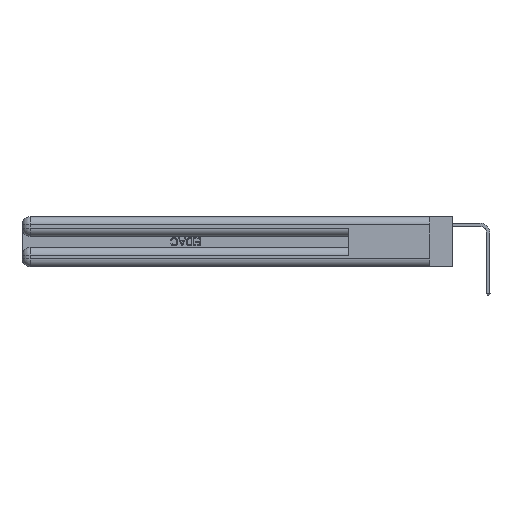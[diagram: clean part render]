
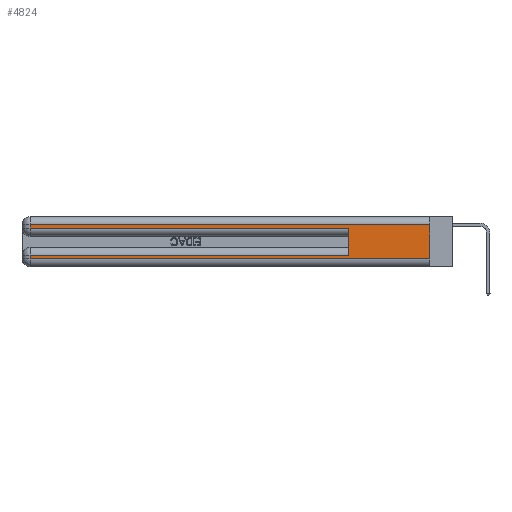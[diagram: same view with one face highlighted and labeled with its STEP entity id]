
A CAD part, left-side view. The second image highlights one B-rep face of the part: STEP entity #4824.
In plain terms, the highlighted planar face has unit normal (-1, 0, 0).
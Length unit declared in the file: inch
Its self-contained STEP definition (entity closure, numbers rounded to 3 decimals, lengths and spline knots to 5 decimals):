
#59 = VECTOR ( 'NONE', #2766, 39.37008 ) ;
#633 = CARTESIAN_POINT ( 'NONE',  ( 0., 0., 0.37 ) ) ;
#1329 = CARTESIAN_POINT ( 'NONE',  ( 0., 0.6, 0.285 ) ) ;
#1531 = VERTEX_POINT ( 'NONE', #12219 ) ;
#1656 = LINE ( 'NONE', #18666, #21440 ) ;
#1940 = DIRECTION ( 'NONE',  ( 0., 0., -1. ) ) ;
#2124 = DIRECTION ( 'NONE',  ( 0., -1., 0. ) ) ;
#2766 = DIRECTION ( 'NONE',  ( 0., 0., -1. ) ) ;
#2821 = CARTESIAN_POINT ( 'NONE',  ( 0., 0., 0.37 ) ) ;
#2968 = DIRECTION ( 'NONE',  ( 0., 0., -1. ) ) ;
#3170 = ORIENTED_EDGE ( 'NONE', *, *, #26253, .T. ) ;
#3863 = DIRECTION ( 'NONE',  ( 0., -1., 0. ) ) ;
#4611 = CARTESIAN_POINT ( 'NONE',  ( 0., 0.6, 0.085 ) ) ;
#4824 = ADVANCED_FACE ( 'NONE', ( #29267 ), #7460, .F. ) ;
#4844 = EDGE_CURVE ( 'NONE', #19728, #23056, #17639, .T. ) ;
#5137 = CARTESIAN_POINT ( 'NONE',  ( 0., 2.94, 0.37 ) ) ;
#5195 = LINE ( 'NONE', #2821, #23765 ) ;
#5652 = CARTESIAN_POINT ( 'NONE',  ( 0., 2.94, 0.06 ) ) ;
#7460 = PLANE ( 'NONE',  #13780 ) ;
#9401 = CARTESIAN_POINT ( 'NONE',  ( 0., 2.94, 0.37 ) ) ;
#9606 = LINE ( 'NONE', #11847, #10082 ) ;
#10082 = VECTOR ( 'NONE', #17260, 39.37008 ) ;
#10135 = VECTOR ( 'NONE', #11826, 39.37008 ) ;
#11091 = EDGE_CURVE ( 'NONE', #17404, #16599, #14023, .T. ) ;
#11424 = CARTESIAN_POINT ( 'NONE',  ( 0., 0., 0.31 ) ) ;
#11826 = DIRECTION ( 'NONE',  ( 0., 0., 1. ) ) ;
#11847 = CARTESIAN_POINT ( 'NONE',  ( 0., 0., 0.085 ) ) ;
#12061 = ORIENTED_EDGE ( 'NONE', *, *, #11091, .T. ) ;
#12219 = CARTESIAN_POINT ( 'NONE',  ( 0., 2.94, 0.285 ) ) ;
#12253 = ORIENTED_EDGE ( 'NONE', *, *, #23209, .T. ) ;
#12267 = ORIENTED_EDGE ( 'NONE', *, *, #4844, .T. ) ;
#12550 = DIRECTION ( 'NONE',  ( 0., 1., 0. ) ) ;
#13015 = DIRECTION ( 'NONE',  ( 1., 0., 0. ) ) ;
#13780 = AXIS2_PLACEMENT_3D ( 'NONE', #633, #13015, #27194 ) ;
#14023 = LINE ( 'NONE', #9401, #26187 ) ;
#14520 = LINE ( 'NONE', #21853, #10135 ) ;
#15435 = CARTESIAN_POINT ( 'NONE',  ( 0., 2.94, 0.085 ) ) ;
#16599 = VERTEX_POINT ( 'NONE', #5652 ) ;
#17260 = DIRECTION ( 'NONE',  ( 0., 1., 0. ) ) ;
#17377 = ORIENTED_EDGE ( 'NONE', *, *, #19979, .F. ) ;
#17404 = VERTEX_POINT ( 'NONE', #15435 ) ;
#17639 = LINE ( 'NONE', #22424, #22937 ) ;
#18430 = VERTEX_POINT ( 'NONE', #1329 ) ;
#18666 = CARTESIAN_POINT ( 'NONE',  ( 0., 0., 0.06 ) ) ;
#18810 = CARTESIAN_POINT ( 'NONE',  ( 0., 0., 0.285 ) ) ;
#19728 = VERTEX_POINT ( 'NONE', #11424 ) ;
#19979 = EDGE_CURVE ( 'NONE', #19728, #23786, #5195, .T. ) ;
#20205 = ORIENTED_EDGE ( 'NONE', *, *, #30081, .T. ) ;
#20667 = CARTESIAN_POINT ( 'NONE',  ( 0., 0., 0.06 ) ) ;
#21191 = LINE ( 'NONE', #18810, #30399 ) ;
#21383 = CARTESIAN_POINT ( 'NONE',  ( 0., 2.94, 0.31 ) ) ;
#21440 = VECTOR ( 'NONE', #2124, 39.37008 ) ;
#21853 = CARTESIAN_POINT ( 'NONE',  ( 0., 0.6, 0.145 ) ) ;
#21926 = EDGE_CURVE ( 'NONE', #27597, #18430, #14520, .T. ) ;
#22424 = CARTESIAN_POINT ( 'NONE',  ( 0., 0., 0.31 ) ) ;
#22937 = VECTOR ( 'NONE', #12550, 39.37008 ) ;
#23056 = VERTEX_POINT ( 'NONE', #21383 ) ;
#23209 = EDGE_CURVE ( 'NONE', #23056, #1531, #26940, .T. ) ;
#23765 = VECTOR ( 'NONE', #2968, 39.37008 ) ;
#23786 = VERTEX_POINT ( 'NONE', #20667 ) ;
#25223 = ORIENTED_EDGE ( 'NONE', *, *, #25890, .T. ) ;
#25890 = EDGE_CURVE ( 'NONE', #27597, #17404, #9606, .T. ) ;
#26187 = VECTOR ( 'NONE', #1940, 39.37008 ) ;
#26253 = EDGE_CURVE ( 'NONE', #1531, #18430, #21191, .T. ) ;
#26940 = LINE ( 'NONE', #5137, #59 ) ;
#27194 = DIRECTION ( 'NONE',  ( 0., 0., -1. ) ) ;
#27597 = VERTEX_POINT ( 'NONE', #4611 ) ;
#27673 = ORIENTED_EDGE ( 'NONE', *, *, #21926, .F. ) ;
#29267 = FACE_OUTER_BOUND ( 'NONE', #30393, .T. ) ;
#30081 = EDGE_CURVE ( 'NONE', #16599, #23786, #1656, .T. ) ;
#30393 = EDGE_LOOP ( 'NONE', ( #17377, #12267, #12253, #3170, #27673, #25223, #12061, #20205 ) ) ;
#30399 = VECTOR ( 'NONE', #3863, 39.37008 ) ;
